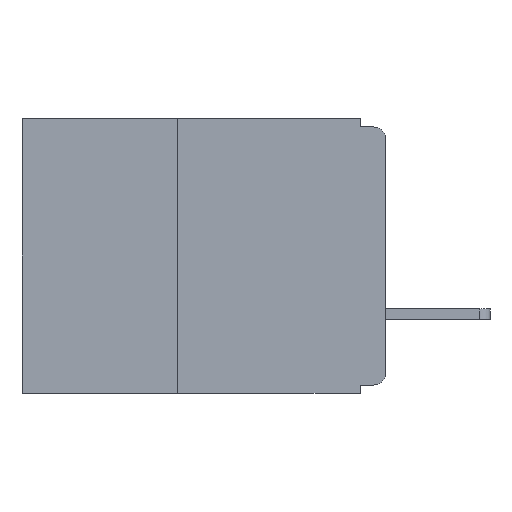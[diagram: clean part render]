
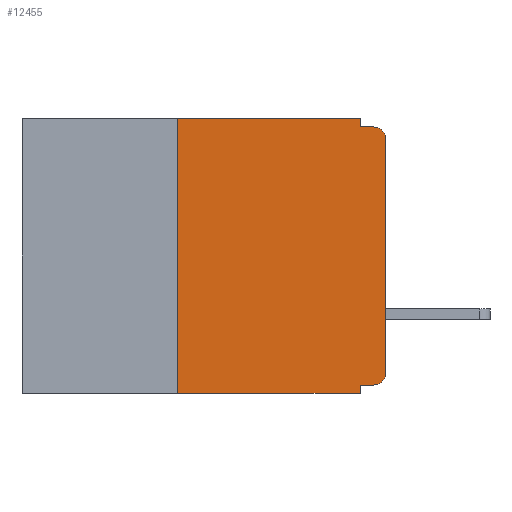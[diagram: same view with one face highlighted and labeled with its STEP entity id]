
A CAD part, left-side view. The second image highlights one B-rep face of the part: STEP entity #12455.
In plain terms, the highlighted planar face has unit normal (-1, 0, 0).
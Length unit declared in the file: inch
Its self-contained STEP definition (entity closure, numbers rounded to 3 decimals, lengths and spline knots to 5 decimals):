
#440 = VECTOR ( 'NONE', #514, 39.37008 ) ;
#514 = DIRECTION ( 'NONE',  ( 0., 0., -1. ) ) ;
#1041 = VECTOR ( 'NONE', #5832, 39.37008 ) ;
#1329 = VERTEX_POINT ( 'NONE', #19122 ) ;
#1678 = DIRECTION ( 'NONE',  ( 0., 0., -1. ) ) ;
#1793 = AXIS2_PLACEMENT_3D ( 'NONE', #16886, #7410, #18424 ) ;
#1943 = EDGE_CURVE ( 'NONE', #3274, #10357, #20240, .T. ) ;
#2012 = VERTEX_POINT ( 'NONE', #15529 ) ;
#2142 = DIRECTION ( 'NONE',  ( 0., 0., 1. ) ) ;
#2296 = DIRECTION ( 'NONE',  ( 0., -1., 0. ) ) ;
#3274 = VERTEX_POINT ( 'NONE', #16625 ) ;
#3965 = VECTOR ( 'NONE', #8984, 39.37008 ) ;
#4267 = EDGE_CURVE ( 'NONE', #10357, #12933, #13018, .T. ) ;
#4315 = CARTESIAN_POINT ( 'NONE',  ( 0., 0.015, -0.32 ) ) ;
#4493 = CARTESIAN_POINT ( 'NONE',  ( 0., 0., -0.32 ) ) ;
#4615 = DIRECTION ( 'NONE',  ( 1., 0., 0. ) ) ;
#4876 = VERTEX_POINT ( 'NONE', #18855 ) ;
#5373 = CIRCLE ( 'NONE', #1793, 0.015 ) ;
#5396 = VECTOR ( 'NONE', #2142, 39.37008 ) ;
#5832 = DIRECTION ( 'NONE',  ( 0., -1., 0. ) ) ;
#6035 = LINE ( 'NONE', #4493, #17686 ) ;
#6128 = ORIENTED_EDGE ( 'NONE', *, *, #6752, .F. ) ;
#6131 = DIRECTION ( 'NONE',  ( 0., 1., 0. ) ) ;
#6752 = EDGE_CURVE ( 'NONE', #19868, #4876, #18518, .T. ) ;
#7053 = VERTEX_POINT ( 'NONE', #9488 ) ;
#7056 = AXIS2_PLACEMENT_3D ( 'NONE', #17860, #8386, #19368 ) ;
#7325 = CARTESIAN_POINT ( 'NONE',  ( 0., 0.437, 0. ) ) ;
#7410 = DIRECTION ( 'NONE',  ( -1., 0., 0. ) ) ;
#7650 = ORIENTED_EDGE ( 'NONE', *, *, #19556, .T. ) ;
#8367 = EDGE_CURVE ( 'NONE', #19964, #12933, #5373, .T. ) ;
#8380 = ORIENTED_EDGE ( 'NONE', *, *, #17678, .T. ) ;
#8386 = DIRECTION ( 'NONE',  ( -1., 0., 0. ) ) ;
#8631 = CARTESIAN_POINT ( 'NONE',  ( 0., 0.031, -0.33 ) ) ;
#8692 = CARTESIAN_POINT ( 'NONE',  ( 0., 0., 0. ) ) ;
#8797 = CIRCLE ( 'NONE', #7056, 0.015 ) ;
#8834 = EDGE_CURVE ( 'NONE', #7053, #1329, #9100, .T. ) ;
#8984 = DIRECTION ( 'NONE',  ( 0., -1., 0. ) ) ;
#9100 = LINE ( 'NONE', #8631, #440 ) ;
#9397 = ORIENTED_EDGE ( 'NONE', *, *, #4267, .F. ) ;
#9488 = CARTESIAN_POINT ( 'NONE',  ( 0., 0.031, -0.32 ) ) ;
#9764 = LINE ( 'NONE', #10397, #10264 ) ;
#10264 = VECTOR ( 'NONE', #2296, 39.37008 ) ;
#10317 = EDGE_CURVE ( 'NONE', #19868, #1329, #9764, .T. ) ;
#10357 = VERTEX_POINT ( 'NONE', #18349 ) ;
#10397 = CARTESIAN_POINT ( 'NONE',  ( 0., 0.437, -0.33 ) ) ;
#10907 = ORIENTED_EDGE ( 'NONE', *, *, #10317, .T. ) ;
#11022 = PLANE ( 'NONE',  #16255 ) ;
#11191 = VECTOR ( 'NONE', #18762, 39.37008 ) ;
#11481 = VECTOR ( 'NONE', #1678, 39.37008 ) ;
#12057 = CARTESIAN_POINT ( 'NONE',  ( 0., 0.031, 0. ) ) ;
#12292 = EDGE_CURVE ( 'NONE', #4876, #3274, #12941, .T. ) ;
#12357 = CARTESIAN_POINT ( 'NONE',  ( 0., 0.25, -0.33 ) ) ;
#12455 = ADVANCED_FACE ( 'NONE', ( #18292 ), #11022, .F. ) ;
#12639 = ORIENTED_EDGE ( 'NONE', *, *, #8367, .T. ) ;
#12933 = VERTEX_POINT ( 'NONE', #17193 ) ;
#12941 = LINE ( 'NONE', #7325, #1041 ) ;
#13018 = LINE ( 'NONE', #17522, #3965 ) ;
#13618 = ORIENTED_EDGE ( 'NONE', *, *, #1943, .F. ) ;
#13879 = LINE ( 'NONE', #8692, #5396 ) ;
#15085 = ORIENTED_EDGE ( 'NONE', *, *, #8834, .F. ) ;
#15529 = CARTESIAN_POINT ( 'NONE',  ( 0., 0., -0.305 ) ) ;
#15581 = ORIENTED_EDGE ( 'NONE', *, *, #19936, .F. ) ;
#15755 = DIRECTION ( 'NONE',  ( 0., 0., -1. ) ) ;
#16101 = VERTEX_POINT ( 'NONE', #4315 ) ;
#16255 = AXIS2_PLACEMENT_3D ( 'NONE', #18806, #4615, #15755 ) ;
#16551 = EDGE_LOOP ( 'NONE', ( #8380, #12639, #9397, #13618, #18251, #6128, #10907, #15085, #15581, #7650 ) ) ;
#16625 = CARTESIAN_POINT ( 'NONE',  ( 0., 0.031, 0. ) ) ;
#16886 = CARTESIAN_POINT ( 'NONE',  ( 0., 0.015, -0.025 ) ) ;
#17193 = CARTESIAN_POINT ( 'NONE',  ( 0., 0.015, -0.01 ) ) ;
#17234 = CARTESIAN_POINT ( 'NONE',  ( 0., 0., -0.025 ) ) ;
#17522 = CARTESIAN_POINT ( 'NONE',  ( 0., 0., -0.01 ) ) ;
#17678 = EDGE_CURVE ( 'NONE', #2012, #19964, #13879, .T. ) ;
#17686 = VECTOR ( 'NONE', #6131, 39.37008 ) ;
#17860 = CARTESIAN_POINT ( 'NONE',  ( 0., 0.015, -0.305 ) ) ;
#18251 = ORIENTED_EDGE ( 'NONE', *, *, #12292, .F. ) ;
#18292 = FACE_OUTER_BOUND ( 'NONE', #16551, .T. ) ;
#18349 = CARTESIAN_POINT ( 'NONE',  ( 0., 0.031, -0.01 ) ) ;
#18424 = DIRECTION ( 'NONE',  ( 0., 0., -1. ) ) ;
#18518 = LINE ( 'NONE', #18764, #11191 ) ;
#18762 = DIRECTION ( 'NONE',  ( 0., 0., 1. ) ) ;
#18764 = CARTESIAN_POINT ( 'NONE',  ( 0., 0.25, -0.33 ) ) ;
#18806 = CARTESIAN_POINT ( 'NONE',  ( 0., 0.437, 0. ) ) ;
#18855 = CARTESIAN_POINT ( 'NONE',  ( 0., 0.25, 0. ) ) ;
#19122 = CARTESIAN_POINT ( 'NONE',  ( 0., 0.031, -0.33 ) ) ;
#19368 = DIRECTION ( 'NONE',  ( 0., 0., -1. ) ) ;
#19556 = EDGE_CURVE ( 'NONE', #16101, #2012, #8797, .T. ) ;
#19868 = VERTEX_POINT ( 'NONE', #12357 ) ;
#19936 = EDGE_CURVE ( 'NONE', #16101, #7053, #6035, .T. ) ;
#19964 = VERTEX_POINT ( 'NONE', #17234 ) ;
#20240 = LINE ( 'NONE', #12057, #11481 ) ;
